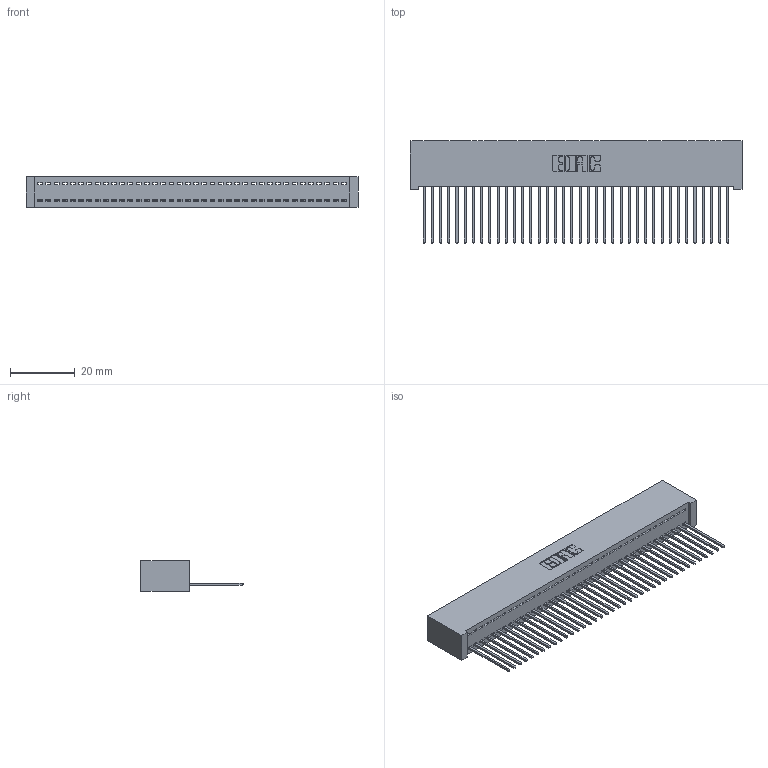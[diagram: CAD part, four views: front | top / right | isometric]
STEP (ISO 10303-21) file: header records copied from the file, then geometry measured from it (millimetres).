
FILE_DESCRIPTION (( 'STEP AP203' ), '1' );
FILE_NAME ('342-038-542-101.STEP', '2018-08-11T22:24:12', ( '' ), ( '' ), 'SwSTEP 2.0', 'SolidWorks 2016', '' );
FILE_SCHEMA (( 'CONFIG_CONTROL_DESIGN' ));
Length unit declared in the file: inch
Products named in the file (3): 342-038-542-101; 342 Part_Lugless; 345-292-001_345-293-142
Assembly tree (39 placements, depth 2):
  342-038-542-101
    342 Part_Lugless
    345-292-001_345-293-142  x38
Bounding box: 102.77 x 31.63 x 9.4 mm (x, y, z)
Volume: 9489.5 mm3; surface area: 14699.2 mm2
Topology: 39 solids, 39 shells, 2306 faces, 6963 edges, 4590 vertices
Faces by surface type: plane 1658, cylinder 648
Entity records: 23357 total; most frequent: CARTESIAN_POINT 4036, ORIENTED_EDGE 4010, DIRECTION 3405, EDGE_CURVE 2005, VECTOR 1885, LINE 1885, VERTEX_POINT 1334, AXIS2_PLACEMENT_3D 760
